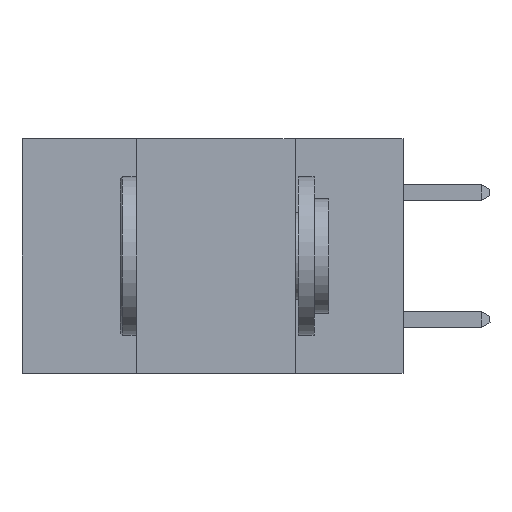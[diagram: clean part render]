
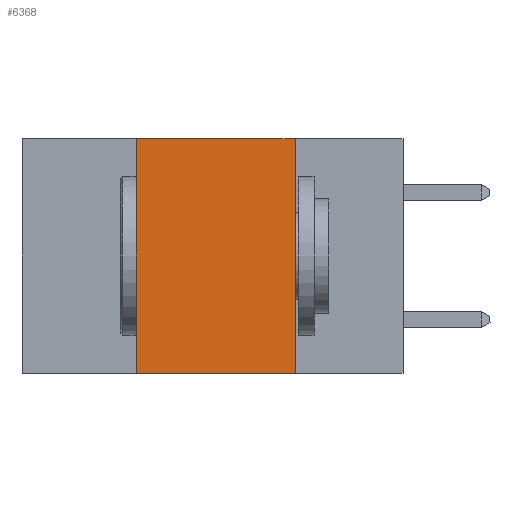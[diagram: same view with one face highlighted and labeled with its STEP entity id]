
A CAD part, left-side view. The second image highlights one B-rep face of the part: STEP entity #6368.
In plain terms, the highlighted planar face has unit normal (-1, 0, 0).
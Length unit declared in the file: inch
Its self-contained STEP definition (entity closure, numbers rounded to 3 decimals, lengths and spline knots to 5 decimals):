
#81 = CARTESIAN_POINT ( 'NONE',  ( 0., 0.17, 0. ) ) ;
#643 = ORIENTED_EDGE ( 'NONE', *, *, #11327, .F. ) ;
#782 = CARTESIAN_POINT ( 'NONE',  ( 0., 0.42, 0. ) ) ;
#958 = DIRECTION ( 'NONE',  ( 0., -1., 0. ) ) ;
#1020 = VERTEX_POINT ( 'NONE', #14089 ) ;
#1906 = DIRECTION ( 'NONE',  ( 0., 0., -1. ) ) ;
#2646 = LINE ( 'NONE', #20141, #18711 ) ;
#4052 = DIRECTION ( 'NONE',  ( 0., 0., 1. ) ) ;
#4364 = CARTESIAN_POINT ( 'NONE',  ( 0., 0.6, 0. ) ) ;
#4581 = VECTOR ( 'NONE', #4052, 39.37008 ) ;
#4690 = ORIENTED_EDGE ( 'NONE', *, *, #20235, .F. ) ;
#4900 = EDGE_CURVE ( 'NONE', #1020, #16749, #5559, .T. ) ;
#5221 = AXIS2_PLACEMENT_3D ( 'NONE', #10699, #18843, #9111 ) ;
#5559 = LINE ( 'NONE', #782, #4581 ) ;
#5931 = DIRECTION ( 'NONE',  ( 0., -1., 0. ) ) ;
#6368 = ADVANCED_FACE ( 'NONE', ( #6716 ), #7551, .F. ) ;
#6375 = CARTESIAN_POINT ( 'NONE',  ( 0., 0.42, 0. ) ) ;
#6716 = FACE_OUTER_BOUND ( 'NONE', #13650, .T. ) ;
#6866 = VECTOR ( 'NONE', #5931, 39.37008 ) ;
#7551 = PLANE ( 'NONE',  #5221 ) ;
#8075 = EDGE_CURVE ( 'NONE', #1020, #9820, #2646, .T. ) ;
#8619 = ORIENTED_EDGE ( 'NONE', *, *, #8075, .T. ) ;
#9111 = DIRECTION ( 'NONE',  ( 0., 0., -1. ) ) ;
#9820 = VERTEX_POINT ( 'NONE', #17943 ) ;
#10699 = CARTESIAN_POINT ( 'NONE',  ( 0., 0.6, 0. ) ) ;
#10988 = ORIENTED_EDGE ( 'NONE', *, *, #4900, .F. ) ;
#11327 = EDGE_CURVE ( 'NONE', #14983, #9820, #17067, .T. ) ;
#11472 = CARTESIAN_POINT ( 'NONE',  ( 0., 0.17, 0. ) ) ;
#11754 = VECTOR ( 'NONE', #1906, 39.37008 ) ;
#13650 = EDGE_LOOP ( 'NONE', ( #643, #4690, #10988, #8619 ) ) ;
#14089 = CARTESIAN_POINT ( 'NONE',  ( 0., 0.42, -0.37 ) ) ;
#14983 = VERTEX_POINT ( 'NONE', #81 ) ;
#16749 = VERTEX_POINT ( 'NONE', #6375 ) ;
#17067 = LINE ( 'NONE', #11472, #11754 ) ;
#17943 = CARTESIAN_POINT ( 'NONE',  ( 0., 0.17, -0.37 ) ) ;
#18711 = VECTOR ( 'NONE', #958, 39.37008 ) ;
#18843 = DIRECTION ( 'NONE',  ( 1., 0., 0. ) ) ;
#19692 = LINE ( 'NONE', #4364, #6866 ) ;
#20141 = CARTESIAN_POINT ( 'NONE',  ( 0., 0.6, -0.37 ) ) ;
#20235 = EDGE_CURVE ( 'NONE', #16749, #14983, #19692, .T. ) ;
